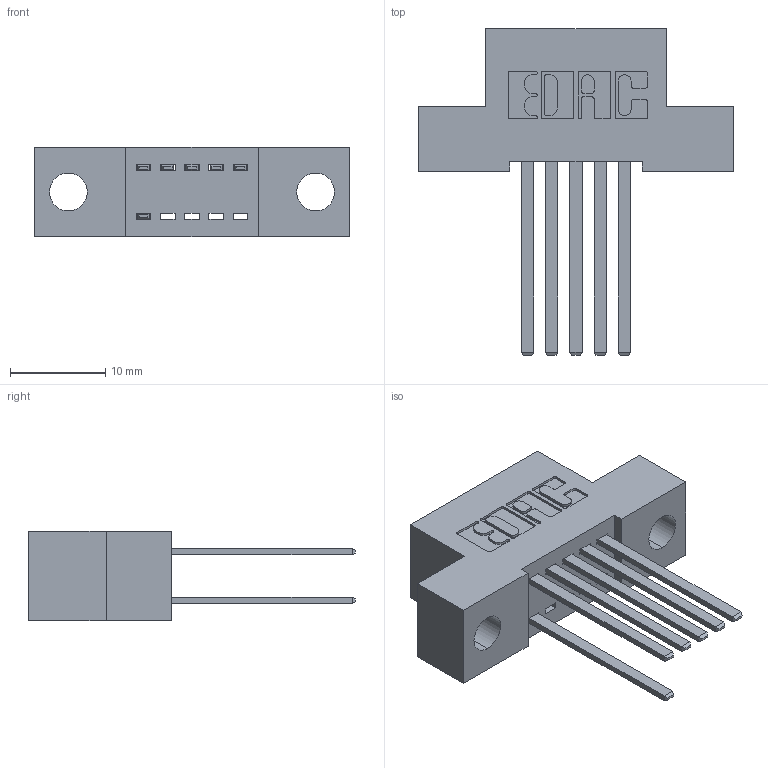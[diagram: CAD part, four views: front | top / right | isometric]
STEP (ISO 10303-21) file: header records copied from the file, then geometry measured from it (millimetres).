
FILE_DESCRIPTION (( 'STEP AP203' ), '1' );
FILE_NAME ('392-010-544-204.STEP', '2018-08-14T20:45:31', ( '' ), ( '' ), 'SwSTEP 2.0', 'SolidWorks 2016', '' );
FILE_SCHEMA (( 'CONFIG_CONTROL_DESIGN' ));
Length unit declared in the file: inch
Products named in the file (3): 342 Part_.156 TH; 345-292-001_345-293-144; 392-010-544-204
Assembly tree (7 placements, depth 2):
  392-010-544-204
    342 Part_.156 TH
    345-292-001_345-293-144  x6
Bounding box: 33.02 x 34.3 x 9.4 mm (x, y, z)
Volume: 2752.8 mm3; surface area: 3427.3 mm2
Topology: 7 solids, 7 shells, 410 faces, 1205 edges, 794 vertices
Faces by surface type: plane 282, cylinder 128
Entity records: 7561 total; most frequent: CARTESIAN_POINT 1310, ORIENTED_EDGE 1250, DIRECTION 1177, EDGE_CURVE 625, VECTOR 501, LINE 501, VERTEX_POINT 414, AXIS2_PLACEMENT_3D 338
